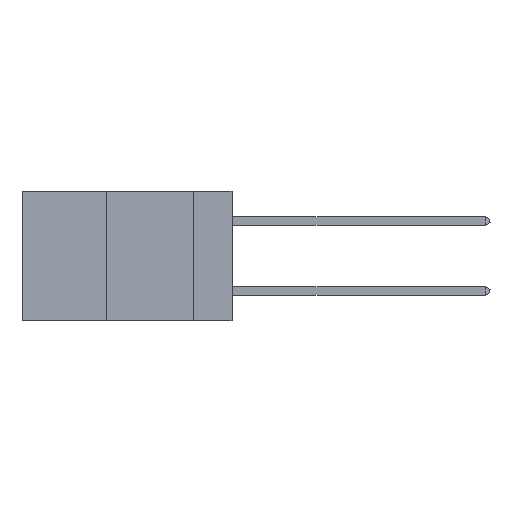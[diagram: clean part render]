
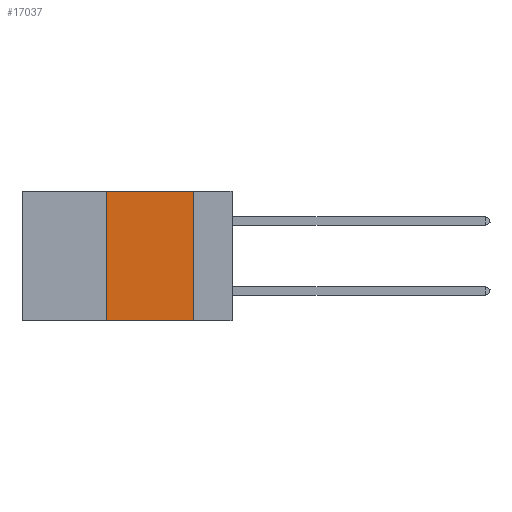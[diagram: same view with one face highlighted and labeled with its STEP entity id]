
A CAD part, left-side view. The second image highlights one B-rep face of the part: STEP entity #17037.
In plain terms, the highlighted planar face has unit normal (-1, 0, 0).
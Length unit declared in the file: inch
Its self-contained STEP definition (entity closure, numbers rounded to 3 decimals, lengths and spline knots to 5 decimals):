
#107 = CARTESIAN_POINT ( 'NONE',  ( 0., 0.6, 0. ) ) ;
#291 = DIRECTION ( 'NONE',  ( 0., 0., -1. ) ) ;
#752 = EDGE_LOOP ( 'NONE', ( #14280, #11085, #15847, #12892 ) ) ;
#2573 = LINE ( 'NONE', #107, #6701 ) ;
#3163 = DIRECTION ( 'NONE',  ( 0., 0., -1. ) ) ;
#4372 = DIRECTION ( 'NONE',  ( 0., -1., 0. ) ) ;
#4448 = DIRECTION ( 'NONE',  ( 0., 0., 1. ) ) ;
#4649 = VERTEX_POINT ( 'NONE', #8238 ) ;
#4875 = CARTESIAN_POINT ( 'NONE',  ( 0., 0.11, 0. ) ) ;
#5131 = VECTOR ( 'NONE', #3163, 39.37008 ) ;
#5231 = EDGE_CURVE ( 'NONE', #4649, #13242, #9761, .T. ) ;
#5787 = CARTESIAN_POINT ( 'NONE',  ( 0., 0.36, 0. ) ) ;
#6701 = VECTOR ( 'NONE', #12433, 39.37008 ) ;
#7167 = EDGE_CURVE ( 'NONE', #19071, #13242, #21374, .T. ) ;
#8238 = CARTESIAN_POINT ( 'NONE',  ( 0., 0.11, 0. ) ) ;
#9065 = CARTESIAN_POINT ( 'NONE',  ( 0., 0.6, 0. ) ) ;
#9624 = FACE_OUTER_BOUND ( 'NONE', #752, .T. ) ;
#9761 = LINE ( 'NONE', #4875, #5131 ) ;
#10817 = DIRECTION ( 'NONE',  ( 1., 0., 0. ) ) ;
#10989 = CARTESIAN_POINT ( 'NONE',  ( 0., 0.36, -0.37 ) ) ;
#11083 = VERTEX_POINT ( 'NONE', #5787 ) ;
#11085 = ORIENTED_EDGE ( 'NONE', *, *, #15174, .F. ) ;
#11336 = LINE ( 'NONE', #16641, #17035 ) ;
#11606 = VECTOR ( 'NONE', #4372, 39.37008 ) ;
#12429 = CARTESIAN_POINT ( 'NONE',  ( 0., 0.11, -0.37 ) ) ;
#12433 = DIRECTION ( 'NONE',  ( 0., -1., 0. ) ) ;
#12892 = ORIENTED_EDGE ( 'NONE', *, *, #7167, .T. ) ;
#13070 = CARTESIAN_POINT ( 'NONE',  ( 0., 0.6, -0.37 ) ) ;
#13242 = VERTEX_POINT ( 'NONE', #12429 ) ;
#14280 = ORIENTED_EDGE ( 'NONE', *, *, #5231, .F. ) ;
#15016 = AXIS2_PLACEMENT_3D ( 'NONE', #9065, #10817, #291 ) ;
#15174 = EDGE_CURVE ( 'NONE', #11083, #4649, #2573, .T. ) ;
#15847 = ORIENTED_EDGE ( 'NONE', *, *, #16062, .F. ) ;
#16062 = EDGE_CURVE ( 'NONE', #19071, #11083, #11336, .T. ) ;
#16641 = CARTESIAN_POINT ( 'NONE',  ( 0., 0.36, 0. ) ) ;
#17035 = VECTOR ( 'NONE', #4448, 39.37008 ) ;
#17037 = ADVANCED_FACE ( 'NONE', ( #9624 ), #19484, .F. ) ;
#19071 = VERTEX_POINT ( 'NONE', #10989 ) ;
#19484 = PLANE ( 'NONE',  #15016 ) ;
#21374 = LINE ( 'NONE', #13070, #11606 ) ;
